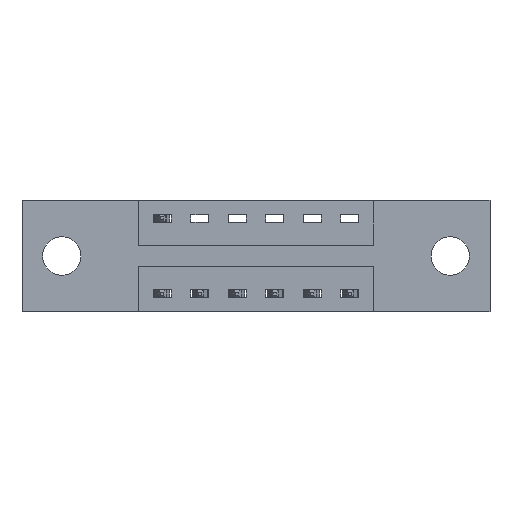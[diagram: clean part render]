
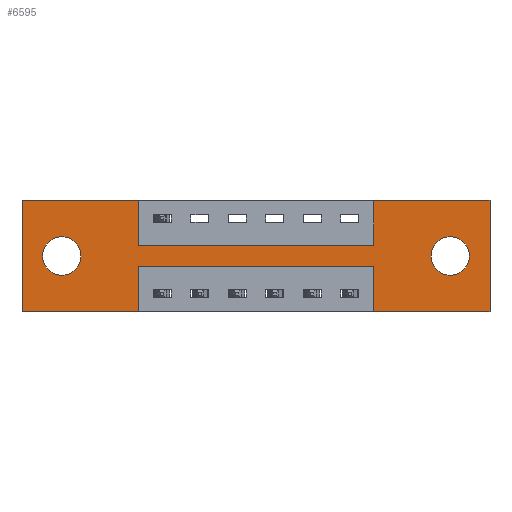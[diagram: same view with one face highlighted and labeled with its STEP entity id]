
A CAD part, front view. The second image highlights one B-rep face of the part: STEP entity #6595.
In plain terms, the highlighted planar face has unit normal (0, -1, 0).
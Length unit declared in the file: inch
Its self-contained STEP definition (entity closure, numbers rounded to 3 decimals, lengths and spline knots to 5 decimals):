
#146 = VERTEX_POINT ( 'NONE', #427 ) ;
#152 = DIRECTION ( 'NONE',  ( 0., 0., 1. ) ) ;
#197 = VECTOR ( 'NONE', #586, 39.37008 ) ;
#205 = CARTESIAN_POINT ( 'NONE',  ( 0.3875, 0., 0. ) ) ;
#245 = CARTESIAN_POINT ( 'NONE',  ( 0., 0., -0.37 ) ) ;
#427 = CARTESIAN_POINT ( 'NONE',  ( 1.1725, 0., -0.37 ) ) ;
#506 = DIRECTION ( 'NONE',  ( 0., 1., 0. ) ) ;
#520 = VERTEX_POINT ( 'NONE', #8630 ) ;
#536 = VECTOR ( 'NONE', #3730, 39.37008 ) ;
#542 = VECTOR ( 'NONE', #7317, 39.37008 ) ;
#586 = DIRECTION ( 'NONE',  ( 1., 0., 0. ) ) ;
#613 = VERTEX_POINT ( 'NONE', #4795 ) ;
#620 = DIRECTION ( 'NONE',  ( 0., 0., 1. ) ) ;
#741 = EDGE_CURVE ( 'NONE', #5275, #8225, #5041, .T. ) ;
#763 = ORIENTED_EDGE ( 'NONE', *, *, #6054, .F. ) ;
#826 = DIRECTION ( 'NONE',  ( -1., 0., 0. ) ) ;
#853 = DIRECTION ( 'NONE',  ( 0., 1., 0. ) ) ;
#867 = ORIENTED_EDGE ( 'NONE', *, *, #8350, .F. ) ;
#868 = VECTOR ( 'NONE', #6716, 39.37008 ) ;
#878 = ORIENTED_EDGE ( 'NONE', *, *, #3707, .T. ) ;
#944 = LINE ( 'NONE', #3415, #7767 ) ;
#975 = AXIS2_PLACEMENT_3D ( 'NONE', #4511, #2521, #7111 ) ;
#1174 = LINE ( 'NONE', #8077, #7988 ) ;
#1199 = PLANE ( 'NONE',  #975 ) ;
#1404 = EDGE_CURVE ( 'NONE', #5246, #613, #6129, .T. ) ;
#1431 = DIRECTION ( 'NONE',  ( 1., 0., 0. ) ) ;
#1505 = DIRECTION ( 'NONE',  ( 0., 1., 0. ) ) ;
#1598 = ORIENTED_EDGE ( 'NONE', *, *, #8055, .F. ) ;
#1690 = ORIENTED_EDGE ( 'NONE', *, *, #6188, .F. ) ;
#1704 = EDGE_CURVE ( 'NONE', #6201, #6455, #5444, .T. ) ;
#1821 = CARTESIAN_POINT ( 'NONE',  ( 0.3875, 0., -0.22 ) ) ;
#1989 = LINE ( 'NONE', #4588, #197 ) ;
#2068 = ORIENTED_EDGE ( 'NONE', *, *, #1404, .F. ) ;
#2082 = VECTOR ( 'NONE', #826, 39.37008 ) ;
#2121 = ORIENTED_EDGE ( 'NONE', *, *, #4051, .T. ) ;
#2216 = ORIENTED_EDGE ( 'NONE', *, *, #6465, .F. ) ;
#2234 = EDGE_CURVE ( 'NONE', #4591, #5246, #1989, .T. ) ;
#2302 = AXIS2_PLACEMENT_3D ( 'NONE', #5483, #1505, #6104 ) ;
#2355 = VERTEX_POINT ( 'NONE', #5388 ) ;
#2365 = LINE ( 'NONE', #245, #7191 ) ;
#2487 = EDGE_CURVE ( 'NONE', #146, #520, #6862, .T. ) ;
#2521 = DIRECTION ( 'NONE',  ( 0., -1., 0. ) ) ;
#2640 = CIRCLE ( 'NONE', #3653, 0.064 ) ;
#2676 = VERTEX_POINT ( 'NONE', #1821 ) ;
#2720 = CARTESIAN_POINT ( 'NONE',  ( 1.1725, 0., 0. ) ) ;
#2864 = VERTEX_POINT ( 'NONE', #6618 ) ;
#2865 = VERTEX_POINT ( 'NONE', #8610 ) ;
#3018 = AXIS2_PLACEMENT_3D ( 'NONE', #7790, #3865, #8466 ) ;
#3124 = FACE_BOUND ( 'NONE', #4101, .T. ) ;
#3287 = ORIENTED_EDGE ( 'NONE', *, *, #4279, .F. ) ;
#3415 = CARTESIAN_POINT ( 'NONE',  ( 0., 0., 0. ) ) ;
#3570 = DIRECTION ( 'NONE',  ( 0., 0., 1. ) ) ;
#3653 = AXIS2_PLACEMENT_3D ( 'NONE', #4859, #853, #5506 ) ;
#3677 = EDGE_CURVE ( 'NONE', #3771, #6720, #7895, .T. ) ;
#3706 = ORIENTED_EDGE ( 'NONE', *, *, #2487, .F. ) ;
#3707 = EDGE_CURVE ( 'NONE', #8225, #5275, #2640, .T. ) ;
#3730 = DIRECTION ( 'NONE',  ( 0., 0., -1. ) ) ;
#3771 = VERTEX_POINT ( 'NONE', #6799 ) ;
#3814 = ORIENTED_EDGE ( 'NONE', *, *, #3677, .T. ) ;
#3865 = DIRECTION ( 'NONE',  ( 0., 1., 0. ) ) ;
#4051 = EDGE_CURVE ( 'NONE', #6720, #3771, #7052, .T. ) ;
#4101 = EDGE_LOOP ( 'NONE', ( #2121, #3814 ) ) ;
#4112 = LINE ( 'NONE', #2720, #542 ) ;
#4173 = VECTOR ( 'NONE', #8333, 39.37008 ) ;
#4186 = CARTESIAN_POINT ( 'NONE',  ( 0.1325, 0., -0.249 ) ) ;
#4247 = VECTOR ( 'NONE', #8599, 39.37008 ) ;
#4278 = CARTESIAN_POINT ( 'NONE',  ( 0.3875, 0., -0.22 ) ) ;
#4279 = EDGE_CURVE ( 'NONE', #2865, #7953, #4112, .T. ) ;
#4319 = ORIENTED_EDGE ( 'NONE', *, *, #741, .T. ) ;
#4454 = CARTESIAN_POINT ( 'NONE',  ( 1.1725, 0., 0. ) ) ;
#4463 = LINE ( 'NONE', #7914, #4247 ) ;
#4466 = AXIS2_PLACEMENT_3D ( 'NONE', #7860, #506, #620 ) ;
#4511 = CARTESIAN_POINT ( 'NONE',  ( 0., 0., -0.37 ) ) ;
#4588 = CARTESIAN_POINT ( 'NONE',  ( 0., 0., 0. ) ) ;
#4591 = VERTEX_POINT ( 'NONE', #7753 ) ;
#4606 = DIRECTION ( 'NONE',  ( 0., 0., -1. ) ) ;
#4795 = CARTESIAN_POINT ( 'NONE',  ( 0.3875, 0., -0.15 ) ) ;
#4859 = CARTESIAN_POINT ( 'NONE',  ( 0.1325, 0., -0.185 ) ) ;
#4994 = CARTESIAN_POINT ( 'NONE',  ( 0.3875, 0., 0. ) ) ;
#5041 = CIRCLE ( 'NONE', #4466, 0.064 ) ;
#5106 = FACE_OUTER_BOUND ( 'NONE', #6388, .T. ) ;
#5115 = VECTOR ( 'NONE', #4606, 39.37008 ) ;
#5161 = VECTOR ( 'NONE', #3570, 39.37008 ) ;
#5246 = VERTEX_POINT ( 'NONE', #4994 ) ;
#5269 = EDGE_LOOP ( 'NONE', ( #4319, #878 ) ) ;
#5275 = VERTEX_POINT ( 'NONE', #7578 ) ;
#5281 = CARTESIAN_POINT ( 'NONE',  ( 1.4275, 0., -0.121 ) ) ;
#5388 = CARTESIAN_POINT ( 'NONE',  ( 0., 0., -0.37 ) ) ;
#5444 = LINE ( 'NONE', #7352, #536 ) ;
#5483 = CARTESIAN_POINT ( 'NONE',  ( 1.4275, 0., -0.185 ) ) ;
#5506 = DIRECTION ( 'NONE',  ( 0., 0., 1. ) ) ;
#5683 = CARTESIAN_POINT ( 'NONE',  ( 1.56, 0., -0.37 ) ) ;
#5686 = EDGE_CURVE ( 'NONE', #2355, #4591, #1174, .T. ) ;
#6033 = CARTESIAN_POINT ( 'NONE',  ( 1.56, 0., 0. ) ) ;
#6054 = EDGE_CURVE ( 'NONE', #2676, #2864, #6822, .T. ) ;
#6104 = DIRECTION ( 'NONE',  ( 0., 0., -1. ) ) ;
#6129 = LINE ( 'NONE', #205, #868 ) ;
#6138 = ORIENTED_EDGE ( 'NONE', *, *, #6351, .F. ) ;
#6188 = EDGE_CURVE ( 'NONE', #7953, #6201, #944, .T. ) ;
#6201 = VERTEX_POINT ( 'NONE', #6033 ) ;
#6323 = CARTESIAN_POINT ( 'NONE',  ( 0.3875, 0., -0.15 ) ) ;
#6351 = EDGE_CURVE ( 'NONE', #520, #2676, #6725, .T. ) ;
#6388 = EDGE_LOOP ( 'NONE', ( #763, #6138, #3706, #1598, #7057, #1690, #3287, #2216, #2068, #7244, #7866, #867 ) ) ;
#6455 = VERTEX_POINT ( 'NONE', #5683 ) ;
#6465 = EDGE_CURVE ( 'NONE', #613, #2865, #7647, .T. ) ;
#6595 = ADVANCED_FACE ( 'NONE', ( #3124, #6616, #5106 ), #1199, .T. ) ;
#6616 = FACE_BOUND ( 'NONE', #5269, .T. ) ;
#6618 = CARTESIAN_POINT ( 'NONE',  ( 0.3875, 0., -0.37 ) ) ;
#6716 = DIRECTION ( 'NONE',  ( 0., 0., -1. ) ) ;
#6720 = VERTEX_POINT ( 'NONE', #5281 ) ;
#6725 = LINE ( 'NONE', #4278, #2082 ) ;
#6799 = CARTESIAN_POINT ( 'NONE',  ( 1.4275, 0., -0.249 ) ) ;
#6822 = LINE ( 'NONE', #7180, #5115 ) ;
#6862 = LINE ( 'NONE', #7493, #5161 ) ;
#7052 = CIRCLE ( 'NONE', #3018, 0.064 ) ;
#7057 = ORIENTED_EDGE ( 'NONE', *, *, #1704, .F. ) ;
#7111 = DIRECTION ( 'NONE',  ( 0., 0., -1. ) ) ;
#7180 = CARTESIAN_POINT ( 'NONE',  ( 0.3875, 0., -0.37 ) ) ;
#7191 = VECTOR ( 'NONE', #8200, 39.37008 ) ;
#7244 = ORIENTED_EDGE ( 'NONE', *, *, #2234, .F. ) ;
#7317 = DIRECTION ( 'NONE',  ( 0., 0., 1. ) ) ;
#7352 = CARTESIAN_POINT ( 'NONE',  ( 1.56, 0., 0. ) ) ;
#7493 = CARTESIAN_POINT ( 'NONE',  ( 1.1725, 0., -0.37 ) ) ;
#7578 = CARTESIAN_POINT ( 'NONE',  ( 0.1325, 0., -0.121 ) ) ;
#7647 = LINE ( 'NONE', #6323, #4173 ) ;
#7753 = CARTESIAN_POINT ( 'NONE',  ( 0., 0., 0. ) ) ;
#7767 = VECTOR ( 'NONE', #1431, 39.37008 ) ;
#7790 = CARTESIAN_POINT ( 'NONE',  ( 1.4275, 0., -0.185 ) ) ;
#7860 = CARTESIAN_POINT ( 'NONE',  ( 0.1325, 0., -0.185 ) ) ;
#7866 = ORIENTED_EDGE ( 'NONE', *, *, #5686, .F. ) ;
#7895 = CIRCLE ( 'NONE', #2302, 0.064 ) ;
#7914 = CARTESIAN_POINT ( 'NONE',  ( 0., 0., -0.37 ) ) ;
#7953 = VERTEX_POINT ( 'NONE', #4454 ) ;
#7988 = VECTOR ( 'NONE', #152, 39.37008 ) ;
#8055 = EDGE_CURVE ( 'NONE', #6455, #146, #4463, .T. ) ;
#8077 = CARTESIAN_POINT ( 'NONE',  ( 0., 0., 0. ) ) ;
#8200 = DIRECTION ( 'NONE',  ( -1., 0., 0. ) ) ;
#8225 = VERTEX_POINT ( 'NONE', #4186 ) ;
#8333 = DIRECTION ( 'NONE',  ( 1., 0., 0. ) ) ;
#8350 = EDGE_CURVE ( 'NONE', #2864, #2355, #2365, .T. ) ;
#8466 = DIRECTION ( 'NONE',  ( 0., 0., -1. ) ) ;
#8599 = DIRECTION ( 'NONE',  ( -1., 0., 0. ) ) ;
#8610 = CARTESIAN_POINT ( 'NONE',  ( 1.1725, 0., -0.15 ) ) ;
#8630 = CARTESIAN_POINT ( 'NONE',  ( 1.1725, 0., -0.22 ) ) ;
